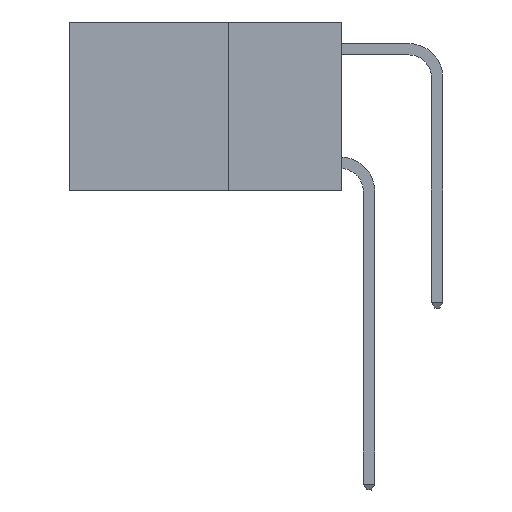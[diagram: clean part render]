
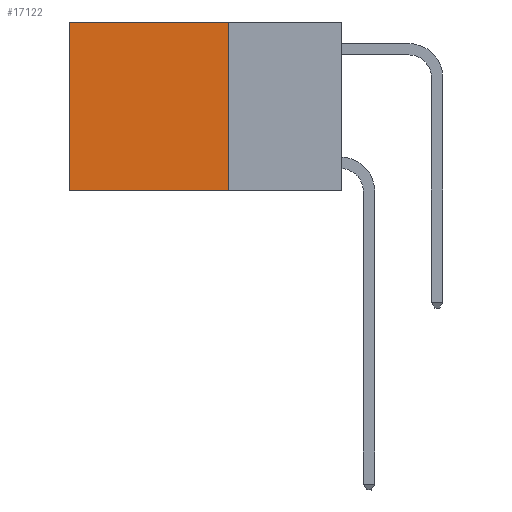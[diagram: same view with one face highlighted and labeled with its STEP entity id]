
A CAD part, left-side view. The second image highlights one B-rep face of the part: STEP entity #17122.
In plain terms, the highlighted planar face has unit normal (-1, 0, 0).
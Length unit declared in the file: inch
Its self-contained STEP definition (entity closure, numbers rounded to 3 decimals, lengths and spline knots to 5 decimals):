
#915 = DIRECTION ( 'NONE',  ( 0., 0., -1. ) ) ;
#1155 = DIRECTION ( 'NONE',  ( 0., 0., -1. ) ) ;
#1379 = VERTEX_POINT ( 'NONE', #5513 ) ;
#1524 = EDGE_CURVE ( 'NONE', #11352, #1379, #7041, .T. ) ;
#2063 = LINE ( 'NONE', #15742, #15834 ) ;
#2523 = ORIENTED_EDGE ( 'NONE', *, *, #8246, .T. ) ;
#3208 = EDGE_LOOP ( 'NONE', ( #2523, #12729, #13783, #16332 ) ) ;
#3999 = VERTEX_POINT ( 'NONE', #16430 ) ;
#4385 = DIRECTION ( 'NONE',  ( 0., 0., -1. ) ) ;
#5513 = CARTESIAN_POINT ( 'NONE',  ( 0.2625, 0.25, -0.37 ) ) ;
#5772 = LINE ( 'NONE', #16290, #9096 ) ;
#6930 = CARTESIAN_POINT ( 'NONE',  ( 0.2625, 0.6, -0.37 ) ) ;
#7041 = LINE ( 'NONE', #11365, #10346 ) ;
#7916 = CARTESIAN_POINT ( 'NONE',  ( 0.2625, 0.25, 0. ) ) ;
#8246 = EDGE_CURVE ( 'NONE', #3999, #8289, #5772, .T. ) ;
#8289 = VERTEX_POINT ( 'NONE', #6930 ) ;
#8859 = DIRECTION ( 'NONE',  ( 0., 1., 0. ) ) ;
#9093 = DIRECTION ( 'NONE',  ( 0., 1., 0. ) ) ;
#9096 = VECTOR ( 'NONE', #1155, 39.37008 ) ;
#9424 = DIRECTION ( 'NONE',  ( 1., 0., 0. ) ) ;
#10346 = VECTOR ( 'NONE', #4385, 39.37008 ) ;
#10878 = LINE ( 'NONE', #16856, #17500 ) ;
#11352 = VERTEX_POINT ( 'NONE', #7916 ) ;
#11365 = CARTESIAN_POINT ( 'NONE',  ( 0.2625, 0.25, 0. ) ) ;
#12729 = ORIENTED_EDGE ( 'NONE', *, *, #13107, .F. ) ;
#13014 = EDGE_CURVE ( 'NONE', #11352, #3999, #10878, .T. ) ;
#13107 = EDGE_CURVE ( 'NONE', #1379, #8289, #2063, .T. ) ;
#13554 = AXIS2_PLACEMENT_3D ( 'NONE', #17390, #9424, #915 ) ;
#13783 = ORIENTED_EDGE ( 'NONE', *, *, #1524, .F. ) ;
#14751 = PLANE ( 'NONE',  #13554 ) ;
#14945 = FACE_OUTER_BOUND ( 'NONE', #3208, .T. ) ;
#15742 = CARTESIAN_POINT ( 'NONE',  ( 0.2625, 0.25, -0.37 ) ) ;
#15834 = VECTOR ( 'NONE', #9093, 39.37008 ) ;
#16290 = CARTESIAN_POINT ( 'NONE',  ( 0.2625, 0.6, 0. ) ) ;
#16332 = ORIENTED_EDGE ( 'NONE', *, *, #13014, .T. ) ;
#16430 = CARTESIAN_POINT ( 'NONE',  ( 0.2625, 0.6, 0. ) ) ;
#16856 = CARTESIAN_POINT ( 'NONE',  ( 0.2625, 0.25, 0. ) ) ;
#17122 = ADVANCED_FACE ( 'NONE', ( #14945 ), #14751, .F. ) ;
#17390 = CARTESIAN_POINT ( 'NONE',  ( 0.2625, 0.25, 0. ) ) ;
#17500 = VECTOR ( 'NONE', #8859, 39.37008 ) ;
